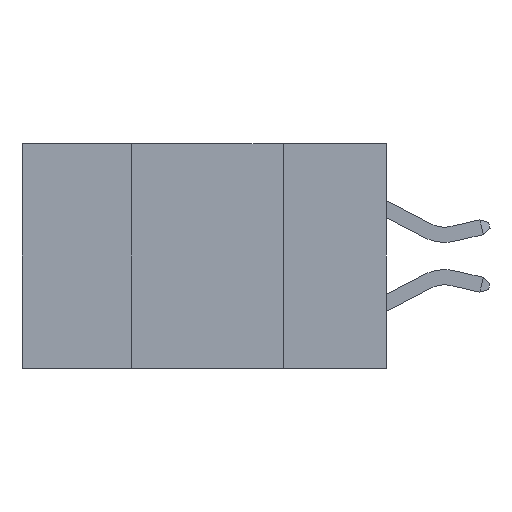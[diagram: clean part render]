
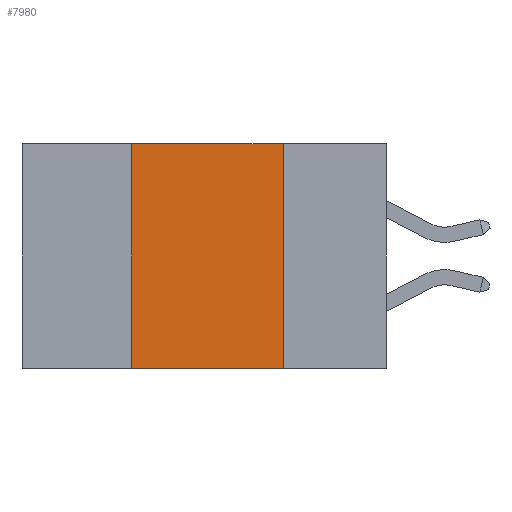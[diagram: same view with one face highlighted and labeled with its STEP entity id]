
A CAD part, left-side view. The second image highlights one B-rep face of the part: STEP entity #7980.
In plain terms, the highlighted planar face has unit normal (-1, 0, 0).
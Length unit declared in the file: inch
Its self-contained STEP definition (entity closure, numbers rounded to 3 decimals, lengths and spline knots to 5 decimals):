
#707 = DIRECTION ( 'NONE',  ( 0., -1., 0. ) ) ;
#774 = VECTOR ( 'NONE', #9987, 39.37008 ) ;
#1305 = ORIENTED_EDGE ( 'NONE', *, *, #7043, .T. ) ;
#1517 = VERTEX_POINT ( 'NONE', #3241 ) ;
#2020 = LINE ( 'NONE', #6262, #13626 ) ;
#2303 = CARTESIAN_POINT ( 'NONE',  ( 0., 0.6, 0. ) ) ;
#2699 = LINE ( 'NONE', #9301, #9120 ) ;
#2746 = ORIENTED_EDGE ( 'NONE', *, *, #5339, .F. ) ;
#3013 = VERTEX_POINT ( 'NONE', #8471 ) ;
#3241 = CARTESIAN_POINT ( 'NONE',  ( 0., 0.17, 0. ) ) ;
#3458 = ORIENTED_EDGE ( 'NONE', *, *, #12772, .F. ) ;
#3483 = DIRECTION ( 'NONE',  ( 0., 0., 1. ) ) ;
#4940 = PLANE ( 'NONE',  #6319 ) ;
#5339 = EDGE_CURVE ( 'NONE', #6885, #1517, #8910, .T. ) ;
#5565 = ORIENTED_EDGE ( 'NONE', *, *, #13446, .F. ) ;
#6160 = DIRECTION ( 'NONE',  ( 0., 0., -1. ) ) ;
#6262 = CARTESIAN_POINT ( 'NONE',  ( 0., 0.6, -0.37 ) ) ;
#6319 = AXIS2_PLACEMENT_3D ( 'NONE', #8298, #12673, #6160 ) ;
#6885 = VERTEX_POINT ( 'NONE', #11566 ) ;
#7043 = EDGE_CURVE ( 'NONE', #12544, #3013, #2020, .T. ) ;
#7304 = FACE_OUTER_BOUND ( 'NONE', #9883, .T. ) ;
#7408 = LINE ( 'NONE', #7475, #10330 ) ;
#7475 = CARTESIAN_POINT ( 'NONE',  ( 0., 0.17, -0.37 ) ) ;
#7980 = ADVANCED_FACE ( 'NONE', ( #7304 ), #4940, .F. ) ;
#8298 = CARTESIAN_POINT ( 'NONE',  ( 0., 0.6, 0. ) ) ;
#8471 = CARTESIAN_POINT ( 'NONE',  ( 0., 0.17, -0.37 ) ) ;
#8542 = DIRECTION ( 'NONE',  ( 0., 0., -1. ) ) ;
#8910 = LINE ( 'NONE', #2303, #774 ) ;
#9120 = VECTOR ( 'NONE', #3483, 39.37008 ) ;
#9196 = CARTESIAN_POINT ( 'NONE',  ( 0., 0.42, -0.37 ) ) ;
#9301 = CARTESIAN_POINT ( 'NONE',  ( 0., 0.42, -0.37 ) ) ;
#9883 = EDGE_LOOP ( 'NONE', ( #3458, #2746, #5565, #1305 ) ) ;
#9987 = DIRECTION ( 'NONE',  ( 0., -1., 0. ) ) ;
#10330 = VECTOR ( 'NONE', #8542, 39.37008 ) ;
#11566 = CARTESIAN_POINT ( 'NONE',  ( 0., 0.42, 0. ) ) ;
#12544 = VERTEX_POINT ( 'NONE', #9196 ) ;
#12673 = DIRECTION ( 'NONE',  ( 1., 0., 0. ) ) ;
#12772 = EDGE_CURVE ( 'NONE', #1517, #3013, #7408, .T. ) ;
#13446 = EDGE_CURVE ( 'NONE', #12544, #6885, #2699, .T. ) ;
#13626 = VECTOR ( 'NONE', #707, 39.37008 ) ;
